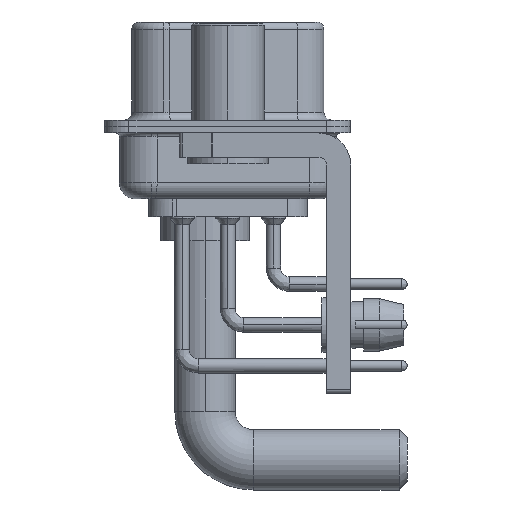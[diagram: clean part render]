
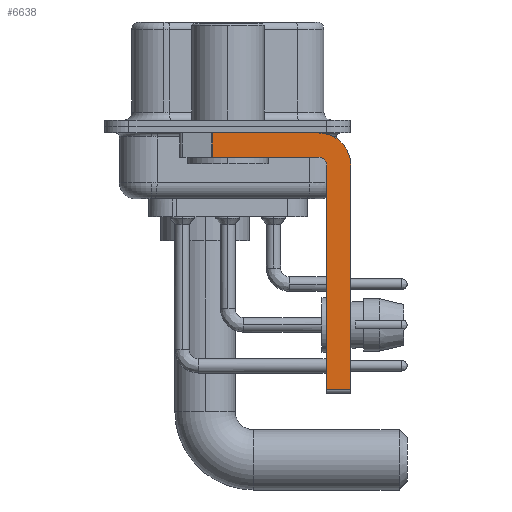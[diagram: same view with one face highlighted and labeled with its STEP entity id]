
A CAD part, left-side view. The second image highlights one B-rep face of the part: STEP entity #6638.
In plain terms, the highlighted planar face has unit normal (-1, 0, 0).
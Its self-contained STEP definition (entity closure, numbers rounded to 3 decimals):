
#54 = DIRECTION ( 'NONE',  ( 0., -1., 0. ) ) ;
#133 = LINE ( 'NONE', #21053, #18161 ) ;
#297 = ORIENTED_EDGE ( 'NONE', *, *, #15774, .F. ) ;
#637 = EDGE_CURVE ( 'NONE', #2525, #3125, #18162, .T. ) ;
#1014 = CARTESIAN_POINT ( 'NONE',  ( -2.9, 0.978, -1.9 ) ) ;
#1268 = EDGE_CURVE ( 'NONE', #38443, #16884, #13081, .T. ) ;
#1540 = ORIENTED_EDGE ( 'NONE', *, *, #17486, .F. ) ;
#2525 = VERTEX_POINT ( 'NONE', #10264 ) ;
#2646 = VERTEX_POINT ( 'NONE', #1014 ) ;
#2682 = EDGE_CURVE ( 'NONE', #3125, #29457, #39267, .T. ) ;
#3125 = VERTEX_POINT ( 'NONE', #7995 ) ;
#4131 = CARTESIAN_POINT ( 'NONE',  ( -2.9, -5.65, -1.9 ) ) ;
#4744 = CARTESIAN_POINT ( 'NONE',  ( -2.9, -7.65, -16.35 ) ) ;
#4917 = DIRECTION ( 'NONE',  ( 0., 0., -1. ) ) ;
#5338 = EDGE_LOOP ( 'NONE', ( #25481, #35977, #297, #1540, #7875, #38490, #23979, #16864 ) ) ;
#6092 = CARTESIAN_POINT ( 'NONE',  ( -2.9, 0.978, -1.9 ) ) ;
#6638 = ADVANCED_FACE ( 'NONE', ( #32472 ), #17364, .F. ) ;
#6656 = CARTESIAN_POINT ( 'NONE',  ( -2.9, -6.15, -16.6 ) ) ;
#6718 = VECTOR ( 'NONE', #7788, 1000. ) ;
#7455 = VERTEX_POINT ( 'NONE', #4744 ) ;
#7788 = DIRECTION ( 'NONE',  ( 0., 0., -1. ) ) ;
#7875 = ORIENTED_EDGE ( 'NONE', *, *, #1268, .F. ) ;
#7995 = CARTESIAN_POINT ( 'NONE',  ( -2.9, -5.65, -0.4 ) ) ;
#8083 = VECTOR ( 'NONE', #18137, 1000. ) ;
#9717 = VECTOR ( 'NONE', #54, 1000. ) ;
#10264 = CARTESIAN_POINT ( 'NONE',  ( -2.9, 0.978, -0.4 ) ) ;
#10909 = AXIS2_PLACEMENT_3D ( 'NONE', #35980, #12045, #39019 ) ;
#10953 = EDGE_CURVE ( 'NONE', #38443, #7455, #133, .T. ) ;
#11051 = DIRECTION ( 'NONE',  ( 1., 0., 0. ) ) ;
#11257 = DIRECTION ( 'NONE',  ( 0., 0., -1. ) ) ;
#12045 = DIRECTION ( 'NONE',  ( -1., 0., 0. ) ) ;
#13081 = LINE ( 'NONE', #6656, #19435 ) ;
#13981 = CARTESIAN_POINT ( 'NONE',  ( -2.9, -5.65, -1.9 ) ) ;
#14138 = DIRECTION ( 'NONE',  ( 1., 0., 0. ) ) ;
#14265 = VERTEX_POINT ( 'NONE', #13981 ) ;
#15774 = EDGE_CURVE ( 'NONE', #14265, #2646, #19593, .T. ) ;
#15816 = CARTESIAN_POINT ( 'NONE',  ( -2.9, -6.15, -16.35 ) ) ;
#16864 = ORIENTED_EDGE ( 'NONE', *, *, #2682, .F. ) ;
#16884 = VERTEX_POINT ( 'NONE', #17809 ) ;
#17364 = PLANE ( 'NONE',  #32040 ) ;
#17486 = EDGE_CURVE ( 'NONE', #16884, #14265, #18623, .T. ) ;
#17809 = CARTESIAN_POINT ( 'NONE',  ( -2.9, -6.15, -2.4 ) ) ;
#18137 = DIRECTION ( 'NONE',  ( 0., 0., -1. ) ) ;
#18161 = VECTOR ( 'NONE', #36744, 1000. ) ;
#18162 = LINE ( 'NONE', #27028, #9717 ) ;
#18623 = CIRCLE ( 'NONE', #10909, 0.5 ) ;
#19435 = VECTOR ( 'NONE', #22533, 1000. ) ;
#19593 = LINE ( 'NONE', #4131, #27510 ) ;
#20188 = CARTESIAN_POINT ( 'NONE',  ( -2.9, -5.65, -2.4 ) ) ;
#21053 = CARTESIAN_POINT ( 'NONE',  ( -2.9, -5.65, -16.35 ) ) ;
#22533 = DIRECTION ( 'NONE',  ( 0., 0., 1. ) ) ;
#23485 = CARTESIAN_POINT ( 'NONE',  ( -2.9, -7.65, -2.4 ) ) ;
#23788 = LINE ( 'NONE', #6092, #8083 ) ;
#23979 = ORIENTED_EDGE ( 'NONE', *, *, #29242, .F. ) ;
#25481 = ORIENTED_EDGE ( 'NONE', *, *, #637, .F. ) ;
#27028 = CARTESIAN_POINT ( 'NONE',  ( -2.9, 3., -0.4 ) ) ;
#27510 = VECTOR ( 'NONE', #28858, 1000. ) ;
#28858 = DIRECTION ( 'NONE',  ( 0., 1., 0. ) ) ;
#29242 = EDGE_CURVE ( 'NONE', #29457, #7455, #31744, .T. ) ;
#29457 = VERTEX_POINT ( 'NONE', #29647 ) ;
#29647 = CARTESIAN_POINT ( 'NONE',  ( -2.9, -7.65, -2.4 ) ) ;
#31575 = EDGE_CURVE ( 'NONE', #2525, #2646, #23788, .T. ) ;
#31744 = LINE ( 'NONE', #23485, #6718 ) ;
#32040 = AXIS2_PLACEMENT_3D ( 'NONE', #20188, #14138, #4917 ) ;
#32472 = FACE_OUTER_BOUND ( 'NONE', #5338, .T. ) ;
#32884 = AXIS2_PLACEMENT_3D ( 'NONE', #38826, #11051, #11257 ) ;
#35977 = ORIENTED_EDGE ( 'NONE', *, *, #31575, .T. ) ;
#35980 = CARTESIAN_POINT ( 'NONE',  ( -2.9, -5.65, -2.4 ) ) ;
#36744 = DIRECTION ( 'NONE',  ( 0., -1., 0. ) ) ;
#38443 = VERTEX_POINT ( 'NONE', #15816 ) ;
#38490 = ORIENTED_EDGE ( 'NONE', *, *, #10953, .T. ) ;
#38826 = CARTESIAN_POINT ( 'NONE',  ( -2.9, -5.65, -2.4 ) ) ;
#39019 = DIRECTION ( 'NONE',  ( 0., 0., 1. ) ) ;
#39267 = CIRCLE ( 'NONE', #32884, 2. ) ;
